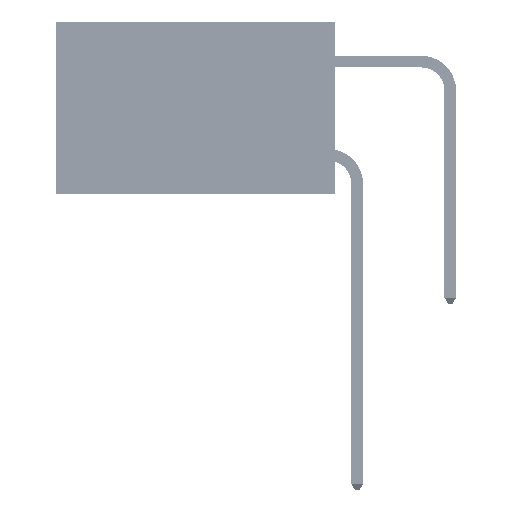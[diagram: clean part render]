
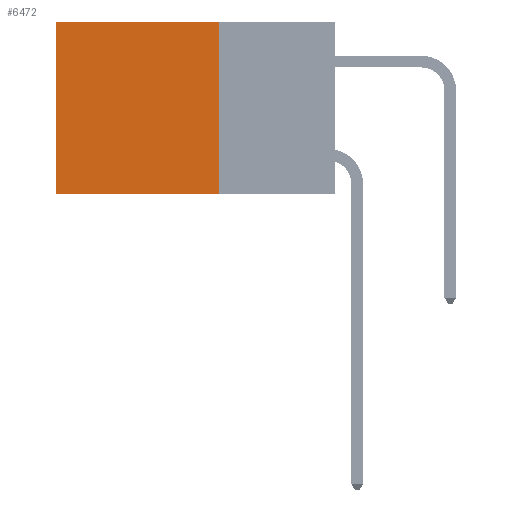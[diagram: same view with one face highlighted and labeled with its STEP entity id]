
A CAD part, left-side view. The second image highlights one B-rep face of the part: STEP entity #6472.
In plain terms, the highlighted planar face has unit normal (-1, 0, 0).
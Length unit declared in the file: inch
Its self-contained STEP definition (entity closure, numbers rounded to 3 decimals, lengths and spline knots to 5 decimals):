
#59 = CARTESIAN_POINT ( 'NONE',  ( 0.2875, 0.6, -0.37 ) ) ;
#3346 = CARTESIAN_POINT ( 'NONE',  ( 0.2875, 0.25, 0. ) ) ;
#3599 = VECTOR ( 'NONE', #16902, 39.37008 ) ;
#4923 = DIRECTION ( 'NONE',  ( 0., 1., 0. ) ) ;
#6443 = DIRECTION ( 'NONE',  ( 0., 1., 0. ) ) ;
#6472 = ADVANCED_FACE ( 'NONE', ( #30612 ), #43090, .F. ) ;
#7030 = DIRECTION ( 'NONE',  ( 0., 0., -1. ) ) ;
#8479 = CARTESIAN_POINT ( 'NONE',  ( 0.2875, 0.6, 0. ) ) ;
#8941 = ORIENTED_EDGE ( 'NONE', *, *, #27503, .F. ) ;
#10583 = LINE ( 'NONE', #41036, #19164 ) ;
#13306 = LINE ( 'NONE', #31270, #3599 ) ;
#14891 = VERTEX_POINT ( 'NONE', #28821 ) ;
#16902 = DIRECTION ( 'NONE',  ( 0., 0., -1. ) ) ;
#17536 = VERTEX_POINT ( 'NONE', #59 ) ;
#19164 = VECTOR ( 'NONE', #4923, 39.37008 ) ;
#22771 = EDGE_CURVE ( 'NONE', #23310, #17536, #13306, .T. ) ;
#22894 = VERTEX_POINT ( 'NONE', #28606 ) ;
#23139 = ORIENTED_EDGE ( 'NONE', *, *, #46242, .T. ) ;
#23310 = VERTEX_POINT ( 'NONE', #8479 ) ;
#26798 = VECTOR ( 'NONE', #42874, 39.37008 ) ;
#27503 = EDGE_CURVE ( 'NONE', #14891, #17536, #30318, .T. ) ;
#28606 = CARTESIAN_POINT ( 'NONE',  ( 0.2875, 0.25, 0. ) ) ;
#28792 = DIRECTION ( 'NONE',  ( 1., 0., 0. ) ) ;
#28821 = CARTESIAN_POINT ( 'NONE',  ( 0.2875, 0.25, -0.37 ) ) ;
#28834 = EDGE_CURVE ( 'NONE', #22894, #14891, #36354, .T. ) ;
#29205 = VECTOR ( 'NONE', #6443, 39.37008 ) ;
#30318 = LINE ( 'NONE', #38899, #29205 ) ;
#30612 = FACE_OUTER_BOUND ( 'NONE', #35946, .T. ) ;
#30724 = AXIS2_PLACEMENT_3D ( 'NONE', #3346, #28792, #7030 ) ;
#31270 = CARTESIAN_POINT ( 'NONE',  ( 0.2875, 0.6, 0. ) ) ;
#31456 = ORIENTED_EDGE ( 'NONE', *, *, #28834, .F. ) ;
#32015 = CARTESIAN_POINT ( 'NONE',  ( 0.2875, 0.25, 0. ) ) ;
#35946 = EDGE_LOOP ( 'NONE', ( #46423, #8941, #31456, #23139 ) ) ;
#36354 = LINE ( 'NONE', #32015, #26798 ) ;
#38899 = CARTESIAN_POINT ( 'NONE',  ( 0.2875, 0.25, -0.37 ) ) ;
#41036 = CARTESIAN_POINT ( 'NONE',  ( 0.2875, 0.25, 0. ) ) ;
#42874 = DIRECTION ( 'NONE',  ( 0., 0., -1. ) ) ;
#43090 = PLANE ( 'NONE',  #30724 ) ;
#46242 = EDGE_CURVE ( 'NONE', #22894, #23310, #10583, .T. ) ;
#46423 = ORIENTED_EDGE ( 'NONE', *, *, #22771, .T. ) ;
